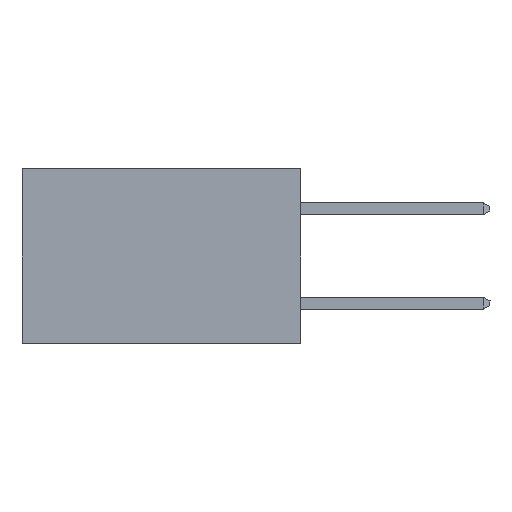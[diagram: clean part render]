
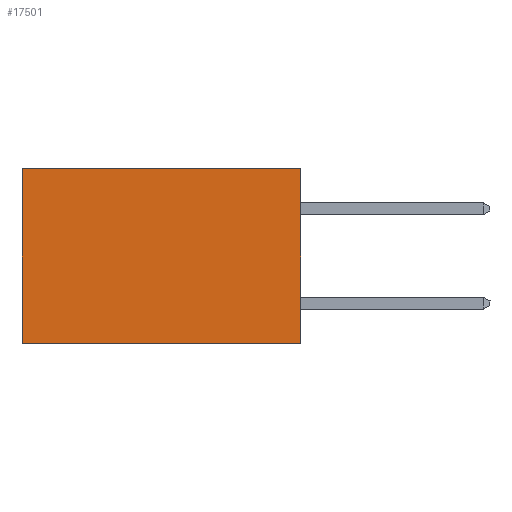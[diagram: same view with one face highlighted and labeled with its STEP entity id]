
A CAD part, left-side view. The second image highlights one B-rep face of the part: STEP entity #17501.
In plain terms, the highlighted planar face has unit normal (-1, 0, 0).
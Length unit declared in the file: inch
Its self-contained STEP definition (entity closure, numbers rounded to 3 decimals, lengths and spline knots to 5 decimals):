
#665 = EDGE_CURVE ( 'NONE', #8496, #2850, #25284, .T. ) ;
#1635 = DIRECTION ( 'NONE',  ( 1., 0., 0. ) ) ;
#2681 = CARTESIAN_POINT ( 'NONE',  ( 0.277, 0.59, -0.37 ) ) ;
#2850 = VERTEX_POINT ( 'NONE', #17744 ) ;
#3405 = VECTOR ( 'NONE', #7945, 39.37008 ) ;
#3625 = CARTESIAN_POINT ( 'NONE',  ( 0.277, 0., 0. ) ) ;
#3723 = LINE ( 'NONE', #19891, #15787 ) ;
#4828 = VERTEX_POINT ( 'NONE', #11431 ) ;
#4843 = EDGE_LOOP ( 'NONE', ( #22675, #24350, #23680, #12286 ) ) ;
#7945 = DIRECTION ( 'NONE',  ( 0., 1., 0. ) ) ;
#8094 = FACE_OUTER_BOUND ( 'NONE', #4843, .T. ) ;
#8496 = VERTEX_POINT ( 'NONE', #3625 ) ;
#11160 = LINE ( 'NONE', #29938, #23649 ) ;
#11431 = CARTESIAN_POINT ( 'NONE',  ( 0.277, 0., -0.37 ) ) ;
#12286 = ORIENTED_EDGE ( 'NONE', *, *, #665, .T. ) ;
#13268 = EDGE_CURVE ( 'NONE', #2850, #25457, #3723, .T. ) ;
#13752 = PLANE ( 'NONE',  #20416 ) ;
#13991 = LINE ( 'NONE', #22131, #3405 ) ;
#15787 = VECTOR ( 'NONE', #22421, 39.37008 ) ;
#15987 = DIRECTION ( 'NONE',  ( 0., 0., -1. ) ) ;
#17501 = ADVANCED_FACE ( 'NONE', ( #8094 ), #13752, .F. ) ;
#17569 = DIRECTION ( 'NONE',  ( 0., 1., 0. ) ) ;
#17744 = CARTESIAN_POINT ( 'NONE',  ( 0.277, 0.59, 0. ) ) ;
#18505 = DIRECTION ( 'NONE',  ( 0., 0., -1. ) ) ;
#18597 = EDGE_CURVE ( 'NONE', #4828, #25457, #13991, .T. ) ;
#19106 = VECTOR ( 'NONE', #17569, 39.37008 ) ;
#19371 = CARTESIAN_POINT ( 'NONE',  ( 0.277, 0., 0. ) ) ;
#19891 = CARTESIAN_POINT ( 'NONE',  ( 0.277, 0.59, -0.37 ) ) ;
#20416 = AXIS2_PLACEMENT_3D ( 'NONE', #30074, #1635, #18505 ) ;
#22131 = CARTESIAN_POINT ( 'NONE',  ( 0.277, 0., -0.37 ) ) ;
#22421 = DIRECTION ( 'NONE',  ( 0., 0., -1. ) ) ;
#22675 = ORIENTED_EDGE ( 'NONE', *, *, #13268, .T. ) ;
#23649 = VECTOR ( 'NONE', #15987, 39.37008 ) ;
#23680 = ORIENTED_EDGE ( 'NONE', *, *, #28529, .F. ) ;
#24350 = ORIENTED_EDGE ( 'NONE', *, *, #18597, .F. ) ;
#25284 = LINE ( 'NONE', #19371, #19106 ) ;
#25457 = VERTEX_POINT ( 'NONE', #2681 ) ;
#28529 = EDGE_CURVE ( 'NONE', #8496, #4828, #11160, .T. ) ;
#29938 = CARTESIAN_POINT ( 'NONE',  ( 0.277, 0., -0.37 ) ) ;
#30074 = CARTESIAN_POINT ( 'NONE',  ( 0.277, 0., -0.37 ) ) ;
